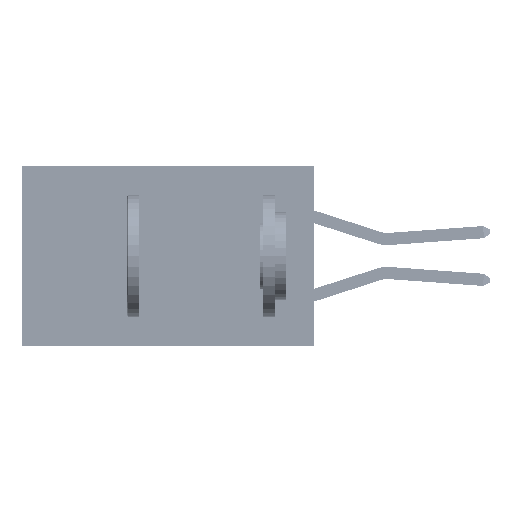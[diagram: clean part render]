
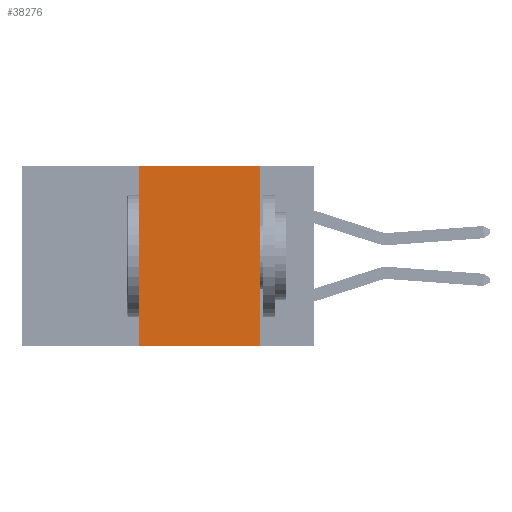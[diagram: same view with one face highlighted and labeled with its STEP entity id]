
A CAD part, left-side view. The second image highlights one B-rep face of the part: STEP entity #38276.
In plain terms, the highlighted planar face has unit normal (-1, 0, 0).
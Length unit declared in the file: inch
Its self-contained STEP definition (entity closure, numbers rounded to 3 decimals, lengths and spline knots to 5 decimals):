
#499 = AXIS2_PLACEMENT_3D ( 'NONE', #4546, #32821, #8391 ) ;
#1629 = DIRECTION ( 'NONE',  ( 0., 0., 1. ) ) ;
#4546 = CARTESIAN_POINT ( 'NONE',  ( 0., 0.6, 0. ) ) ;
#4775 = LINE ( 'NONE', #40488, #9182 ) ;
#4845 = EDGE_CURVE ( 'NONE', #35164, #28388, #32949, .T. ) ;
#6385 = LINE ( 'NONE', #31850, #36633 ) ;
#8128 = ORIENTED_EDGE ( 'NONE', *, *, #16115, .T. ) ;
#8134 = CARTESIAN_POINT ( 'NONE',  ( 0., 0.36, 0. ) ) ;
#8391 = DIRECTION ( 'NONE',  ( 0., 0., -1. ) ) ;
#9182 = VECTOR ( 'NONE', #19882, 39.37008 ) ;
#11831 = CARTESIAN_POINT ( 'NONE',  ( 0., 0.36, -0.37 ) ) ;
#12584 = VERTEX_POINT ( 'NONE', #11831 ) ;
#16115 = EDGE_CURVE ( 'NONE', #12584, #35682, #4775, .T. ) ;
#17032 = VECTOR ( 'NONE', #18314, 39.37008 ) ;
#17549 = CARTESIAN_POINT ( 'NONE',  ( 0., 0.11, -0.37 ) ) ;
#18314 = DIRECTION ( 'NONE',  ( 0., -1., 0. ) ) ;
#19882 = DIRECTION ( 'NONE',  ( 0., -1., 0. ) ) ;
#21713 = CARTESIAN_POINT ( 'NONE',  ( 0., 0.6, 0. ) ) ;
#21850 = DIRECTION ( 'NONE',  ( 0., 0., -1. ) ) ;
#22365 = PLANE ( 'NONE',  #499 ) ;
#24786 = ORIENTED_EDGE ( 'NONE', *, *, #4845, .F. ) ;
#28254 = ORIENTED_EDGE ( 'NONE', *, *, #33637, .F. ) ;
#28388 = VERTEX_POINT ( 'NONE', #42176 ) ;
#30144 = FACE_OUTER_BOUND ( 'NONE', #43938, .T. ) ;
#31850 = CARTESIAN_POINT ( 'NONE',  ( 0., 0.11, 0. ) ) ;
#32821 = DIRECTION ( 'NONE',  ( 1., 0., 0. ) ) ;
#32949 = LINE ( 'NONE', #21713, #17032 ) ;
#33196 = VECTOR ( 'NONE', #1629, 39.37008 ) ;
#33637 = EDGE_CURVE ( 'NONE', #28388, #35682, #6385, .T. ) ;
#34667 = EDGE_CURVE ( 'NONE', #12584, #35164, #42517, .T. ) ;
#35164 = VERTEX_POINT ( 'NONE', #42479 ) ;
#35682 = VERTEX_POINT ( 'NONE', #17549 ) ;
#36633 = VECTOR ( 'NONE', #21850, 39.37008 ) ;
#38276 = ADVANCED_FACE ( 'NONE', ( #30144 ), #22365, .F. ) ;
#38550 = ORIENTED_EDGE ( 'NONE', *, *, #34667, .F. ) ;
#40488 = CARTESIAN_POINT ( 'NONE',  ( 0., 0.6, -0.37 ) ) ;
#42176 = CARTESIAN_POINT ( 'NONE',  ( 0., 0.11, 0. ) ) ;
#42479 = CARTESIAN_POINT ( 'NONE',  ( 0., 0.36, 0. ) ) ;
#42517 = LINE ( 'NONE', #8134, #33196 ) ;
#43938 = EDGE_LOOP ( 'NONE', ( #28254, #24786, #38550, #8128 ) ) ;
